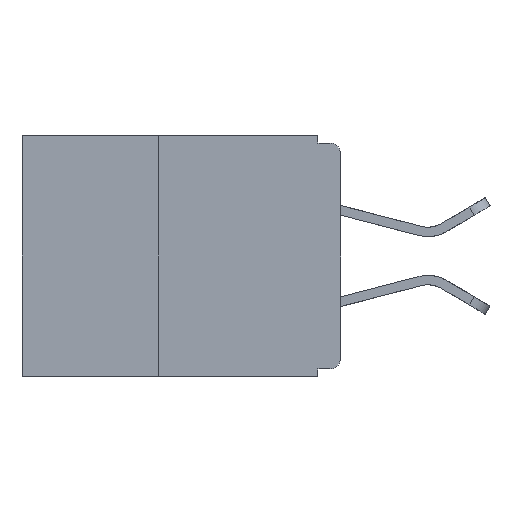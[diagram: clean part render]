
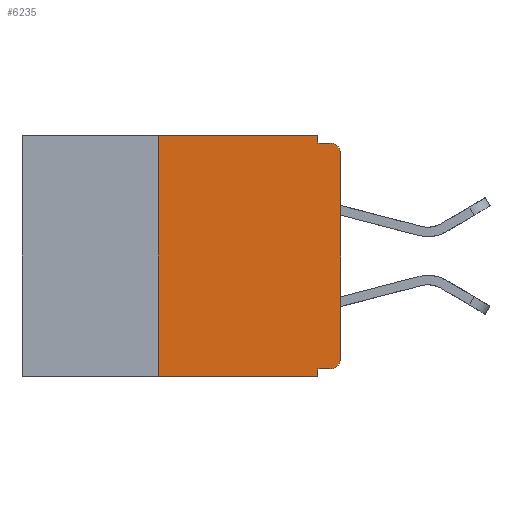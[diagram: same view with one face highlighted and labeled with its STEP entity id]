
A CAD part, left-side view. The second image highlights one B-rep face of the part: STEP entity #6235.
In plain terms, the highlighted planar face has unit normal (-1, 0, 0).
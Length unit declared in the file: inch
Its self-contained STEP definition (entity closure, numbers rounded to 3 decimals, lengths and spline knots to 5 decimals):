
#956 = CIRCLE ( 'NONE', #12862, 0.015 ) ;
#1397 = DIRECTION ( 'NONE',  ( 1., 0., 0. ) ) ;
#1984 = VERTEX_POINT ( 'NONE', #12223 ) ;
#2159 = LINE ( 'NONE', #12829, #29424 ) ;
#2319 = DIRECTION ( 'NONE',  ( 0., -1., 0. ) ) ;
#3811 = CARTESIAN_POINT ( 'NONE',  ( 0., 0.25, -0.33 ) ) ;
#4775 = DIRECTION ( 'NONE',  ( 0., 0., -1. ) ) ;
#5300 = EDGE_LOOP ( 'NONE', ( #27957, #28062, #28384, #28976, #29033, #29156, #29956, #30095, #31056, #31387 ) ) ;
#5459 = EDGE_CURVE ( 'NONE', #25447, #8361, #16886, .T. ) ;
#5568 = CARTESIAN_POINT ( 'NONE',  ( 0., 0., -0.01 ) ) ;
#5656 = LINE ( 'NONE', #9307, #18904 ) ;
#5854 = EDGE_CURVE ( 'NONE', #6950, #26672, #11159, .T. ) ;
#6059 = EDGE_CURVE ( 'NONE', #28153, #1984, #18545, .T. ) ;
#6235 = ADVANCED_FACE ( 'NONE', ( #26727 ), #14644, .F. ) ;
#6338 = EDGE_CURVE ( 'NONE', #31427, #28153, #17288, .T. ) ;
#6394 = CARTESIAN_POINT ( 'NONE',  ( 0., 0.015, -0.305 ) ) ;
#6443 = VERTEX_POINT ( 'NONE', #15569 ) ;
#6741 = DIRECTION ( 'NONE',  ( -1., 0., 0. ) ) ;
#6859 = EDGE_CURVE ( 'NONE', #8361, #11962, #21749, .T. ) ;
#6950 = VERTEX_POINT ( 'NONE', #25477 ) ;
#7122 = CARTESIAN_POINT ( 'NONE',  ( 0., 0.25, -0.33 ) ) ;
#8134 = CARTESIAN_POINT ( 'NONE',  ( 0., 0., 0. ) ) ;
#8361 = VERTEX_POINT ( 'NONE', #25323 ) ;
#8593 = CARTESIAN_POINT ( 'NONE',  ( 0., 0.015, -0.01 ) ) ;
#9037 = VECTOR ( 'NONE', #10810, 39.37008 ) ;
#9053 = DIRECTION ( 'NONE',  ( 0., 0., -1. ) ) ;
#9270 = EDGE_CURVE ( 'NONE', #6443, #11962, #12363, .T. ) ;
#9307 = CARTESIAN_POINT ( 'NONE',  ( 0., 0.437, -0.33 ) ) ;
#9447 = EDGE_CURVE ( 'NONE', #28857, #25447, #956, .T. ) ;
#10796 = LINE ( 'NONE', #25889, #24744 ) ;
#10810 = DIRECTION ( 'NONE',  ( 0., 0., 1. ) ) ;
#11159 = LINE ( 'NONE', #27985, #24269 ) ;
#11563 = VECTOR ( 'NONE', #2319, 39.37008 ) ;
#11816 = CARTESIAN_POINT ( 'NONE',  ( 0., 0., -0.305 ) ) ;
#11962 = VERTEX_POINT ( 'NONE', #8593 ) ;
#12223 = CARTESIAN_POINT ( 'NONE',  ( 0., 0.031, 0. ) ) ;
#12363 = LINE ( 'NONE', #5568, #26313 ) ;
#12829 = CARTESIAN_POINT ( 'NONE',  ( 0., 0., -0.32 ) ) ;
#12862 = AXIS2_PLACEMENT_3D ( 'NONE', #6394, #24803, #9053 ) ;
#13999 = CARTESIAN_POINT ( 'NONE',  ( 0., 0.25, 0. ) ) ;
#14644 = PLANE ( 'NONE',  #30521 ) ;
#14949 = DIRECTION ( 'NONE',  ( 0., 0., -1. ) ) ;
#15465 = DIRECTION ( 'NONE',  ( 0., 1., 0. ) ) ;
#15569 = CARTESIAN_POINT ( 'NONE',  ( 0., 0.031, -0.01 ) ) ;
#16462 = VECTOR ( 'NONE', #33346, 39.37008 ) ;
#16886 = LINE ( 'NONE', #8134, #9037 ) ;
#17053 = CARTESIAN_POINT ( 'NONE',  ( 0., 0.015, -0.32 ) ) ;
#17258 = DIRECTION ( 'NONE',  ( 0., -1., 0. ) ) ;
#17288 = LINE ( 'NONE', #7122, #16462 ) ;
#18013 = CARTESIAN_POINT ( 'NONE',  ( 0., 0.031, -0.33 ) ) ;
#18264 = CARTESIAN_POINT ( 'NONE',  ( 0., 0.437, 0. ) ) ;
#18545 = LINE ( 'NONE', #18264, #11563 ) ;
#18904 = VECTOR ( 'NONE', #17258, 39.37008 ) ;
#20040 = DIRECTION ( 'NONE',  ( 0., 0., -1. ) ) ;
#21645 = EDGE_CURVE ( 'NONE', #31427, #26672, #5656, .T. ) ;
#21749 = CIRCLE ( 'NONE', #29223, 0.015 ) ;
#22486 = CARTESIAN_POINT ( 'NONE',  ( 0., 0.015, -0.025 ) ) ;
#23132 = EDGE_CURVE ( 'NONE', #28857, #6950, #2159, .T. ) ;
#24269 = VECTOR ( 'NONE', #14949, 39.37008 ) ;
#24744 = VECTOR ( 'NONE', #4775, 39.37008 ) ;
#24803 = DIRECTION ( 'NONE',  ( -1., 0., 0. ) ) ;
#25143 = DIRECTION ( 'NONE',  ( 0., 0., -1. ) ) ;
#25323 = CARTESIAN_POINT ( 'NONE',  ( 0., 0., -0.025 ) ) ;
#25447 = VERTEX_POINT ( 'NONE', #11816 ) ;
#25477 = CARTESIAN_POINT ( 'NONE',  ( 0., 0.031, -0.32 ) ) ;
#25713 = EDGE_CURVE ( 'NONE', #1984, #6443, #10796, .T. ) ;
#25889 = CARTESIAN_POINT ( 'NONE',  ( 0., 0.031, 0. ) ) ;
#26313 = VECTOR ( 'NONE', #31767, 39.37008 ) ;
#26672 = VERTEX_POINT ( 'NONE', #18013 ) ;
#26727 = FACE_OUTER_BOUND ( 'NONE', #5300, .T. ) ;
#27957 = ORIENTED_EDGE ( 'NONE', *, *, #5459, .T. ) ;
#27985 = CARTESIAN_POINT ( 'NONE',  ( 0., 0.031, -0.33 ) ) ;
#28062 = ORIENTED_EDGE ( 'NONE', *, *, #6859, .T. ) ;
#28153 = VERTEX_POINT ( 'NONE', #13999 ) ;
#28384 = ORIENTED_EDGE ( 'NONE', *, *, #9270, .F. ) ;
#28857 = VERTEX_POINT ( 'NONE', #17053 ) ;
#28976 = ORIENTED_EDGE ( 'NONE', *, *, #25713, .F. ) ;
#29033 = ORIENTED_EDGE ( 'NONE', *, *, #6059, .F. ) ;
#29156 = ORIENTED_EDGE ( 'NONE', *, *, #6338, .F. ) ;
#29223 = AXIS2_PLACEMENT_3D ( 'NONE', #22486, #6741, #25143 ) ;
#29424 = VECTOR ( 'NONE', #15465, 39.37008 ) ;
#29956 = ORIENTED_EDGE ( 'NONE', *, *, #21645, .T. ) ;
#30095 = ORIENTED_EDGE ( 'NONE', *, *, #5854, .F. ) ;
#30413 = CARTESIAN_POINT ( 'NONE',  ( 0., 0.437, 0. ) ) ;
#30521 = AXIS2_PLACEMENT_3D ( 'NONE', #30413, #1397, #20040 ) ;
#31056 = ORIENTED_EDGE ( 'NONE', *, *, #23132, .F. ) ;
#31387 = ORIENTED_EDGE ( 'NONE', *, *, #9447, .T. ) ;
#31427 = VERTEX_POINT ( 'NONE', #3811 ) ;
#31767 = DIRECTION ( 'NONE',  ( 0., -1., 0. ) ) ;
#33346 = DIRECTION ( 'NONE',  ( 0., 0., 1. ) ) ;
